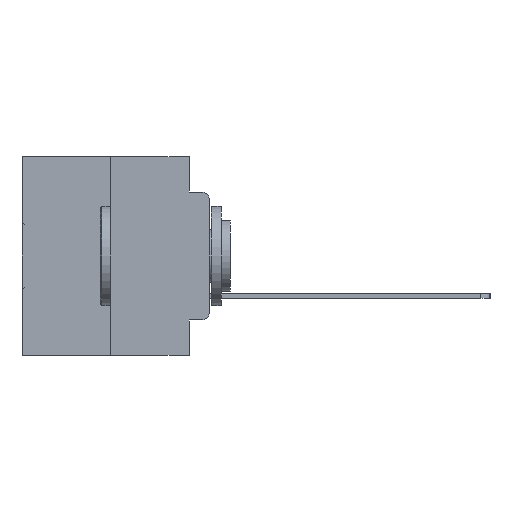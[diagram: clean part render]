
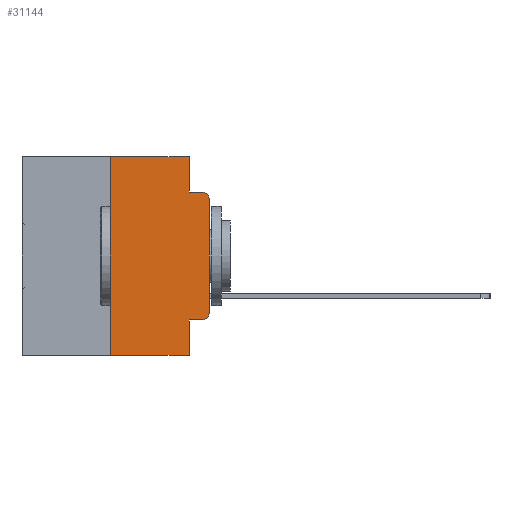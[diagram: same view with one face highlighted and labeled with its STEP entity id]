
A CAD part, left-side view. The second image highlights one B-rep face of the part: STEP entity #31144.
In plain terms, the highlighted planar face has unit normal (-1, 0, 0).
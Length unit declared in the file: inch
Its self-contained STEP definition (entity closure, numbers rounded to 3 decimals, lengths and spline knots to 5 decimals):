
#53 = LINE ( 'NONE', #8204, #6582 ) ;
#226 = CARTESIAN_POINT ( 'NONE',  ( 0., 0.051, -0.4115 ) ) ;
#747 = ORIENTED_EDGE ( 'NONE', *, *, #30713, .F. ) ;
#1232 = CARTESIAN_POINT ( 'NONE',  ( 0., 0.051, -0.0885 ) ) ;
#1269 = DIRECTION ( 'NONE',  ( 0., 0., -1. ) ) ;
#1496 = LINE ( 'NONE', #15368, #13036 ) ;
#2248 = ORIENTED_EDGE ( 'NONE', *, *, #18684, .T. ) ;
#2343 = CARTESIAN_POINT ( 'NONE',  ( 0., 0.02, -0.3915 ) ) ;
#2487 = VERTEX_POINT ( 'NONE', #26427 ) ;
#2679 = DIRECTION ( 'NONE',  ( 0., -1., 0. ) ) ;
#2840 = EDGE_CURVE ( 'NONE', #14777, #12980, #29415, .T. ) ;
#3729 = LINE ( 'NONE', #226, #22547 ) ;
#3903 = DIRECTION ( 'NONE',  ( 0., 0., -1. ) ) ;
#4452 = CARTESIAN_POINT ( 'NONE',  ( 0., 0.25, 0. ) ) ;
#4597 = DIRECTION ( 'NONE',  ( 0., 0., 1. ) ) ;
#4826 = DIRECTION ( 'NONE',  ( 0., 0., -1. ) ) ;
#5545 = EDGE_CURVE ( 'NONE', #18597, #29442, #30926, .T. ) ;
#5785 = ORIENTED_EDGE ( 'NONE', *, *, #19905, .T. ) ;
#6006 = VERTEX_POINT ( 'NONE', #20141 ) ;
#6008 = FACE_OUTER_BOUND ( 'NONE', #26589, .T. ) ;
#6169 = VERTEX_POINT ( 'NONE', #1232 ) ;
#6359 = LINE ( 'NONE', #21562, #18630 ) ;
#6582 = VECTOR ( 'NONE', #15618, 39.37008 ) ;
#6630 = AXIS2_PLACEMENT_3D ( 'NONE', #2343, #19522, #4826 ) ;
#6687 = VECTOR ( 'NONE', #18838, 39.37008 ) ;
#6896 = DIRECTION ( 'NONE',  ( 0., -1., 0. ) ) ;
#6928 = ORIENTED_EDGE ( 'NONE', *, *, #2840, .F. ) ;
#6996 = DIRECTION ( 'NONE',  ( 0., -1., 0. ) ) ;
#8204 = CARTESIAN_POINT ( 'NONE',  ( 0., 0.051, 0. ) ) ;
#8409 = EDGE_CURVE ( 'NONE', #2487, #21073, #9040, .T. ) ;
#8840 = ORIENTED_EDGE ( 'NONE', *, *, #9459, .F. ) ;
#9004 = CARTESIAN_POINT ( 'NONE',  ( 0., 0.473, 0. ) ) ;
#9040 = CIRCLE ( 'NONE', #6630, 0.02 ) ;
#9209 = ORIENTED_EDGE ( 'NONE', *, *, #5545, .T. ) ;
#9459 = EDGE_CURVE ( 'NONE', #28453, #6169, #18917, .T. ) ;
#10090 = CARTESIAN_POINT ( 'NONE',  ( 0., 0., -0.1085 ) ) ;
#11153 = DIRECTION ( 'NONE',  ( -1., 0., 0. ) ) ;
#12410 = VECTOR ( 'NONE', #3903, 39.37008 ) ;
#12980 = VERTEX_POINT ( 'NONE', #19435 ) ;
#13036 = VECTOR ( 'NONE', #27517, 39.37008 ) ;
#13221 = LINE ( 'NONE', #9004, #6687 ) ;
#13465 = ORIENTED_EDGE ( 'NONE', *, *, #30757, .T. ) ;
#14777 = VERTEX_POINT ( 'NONE', #15830 ) ;
#15368 = CARTESIAN_POINT ( 'NONE',  ( 0., 0., 0. ) ) ;
#15618 = DIRECTION ( 'NONE',  ( 0., 0., -1. ) ) ;
#15830 = CARTESIAN_POINT ( 'NONE',  ( 0., 0.25, -0.5 ) ) ;
#16004 = EDGE_CURVE ( 'NONE', #12980, #28453, #13221, .T. ) ;
#16005 = DIRECTION ( 'NONE',  ( 1., 0., 0. ) ) ;
#18221 = VERTEX_POINT ( 'NONE', #20937 ) ;
#18597 = VERTEX_POINT ( 'NONE', #10090 ) ;
#18630 = VECTOR ( 'NONE', #6896, 39.37008 ) ;
#18684 = EDGE_CURVE ( 'NONE', #21073, #18597, #1496, .T. ) ;
#18815 = ORIENTED_EDGE ( 'NONE', *, *, #8409, .T. ) ;
#18838 = DIRECTION ( 'NONE',  ( 0., -1., 0. ) ) ;
#18917 = LINE ( 'NONE', #25888, #12410 ) ;
#19435 = CARTESIAN_POINT ( 'NONE',  ( 0., 0.25, 0. ) ) ;
#19522 = DIRECTION ( 'NONE',  ( -1., 0., 0. ) ) ;
#19905 = EDGE_CURVE ( 'NONE', #18221, #2487, #3729, .T. ) ;
#20141 = CARTESIAN_POINT ( 'NONE',  ( 0., 0.051, -0.5 ) ) ;
#20735 = ORIENTED_EDGE ( 'NONE', *, *, #26474, .F. ) ;
#20937 = CARTESIAN_POINT ( 'NONE',  ( 0., 0.051, -0.4115 ) ) ;
#21073 = VERTEX_POINT ( 'NONE', #21825 ) ;
#21562 = CARTESIAN_POINT ( 'NONE',  ( 0., 0.051, -0.0885 ) ) ;
#21825 = CARTESIAN_POINT ( 'NONE',  ( 0., 0., -0.3915 ) ) ;
#22281 = CARTESIAN_POINT ( 'NONE',  ( 0., 0.02, -0.0885 ) ) ;
#22547 = VECTOR ( 'NONE', #2679, 39.37008 ) ;
#22764 = CARTESIAN_POINT ( 'NONE',  ( 0., 0.051, 0. ) ) ;
#22968 = VECTOR ( 'NONE', #4597, 39.37008 ) ;
#24146 = CARTESIAN_POINT ( 'NONE',  ( 0., 0.473, -0.5 ) ) ;
#24244 = AXIS2_PLACEMENT_3D ( 'NONE', #25834, #11153, #28249 ) ;
#24400 = LINE ( 'NONE', #24146, #31560 ) ;
#25272 = AXIS2_PLACEMENT_3D ( 'NONE', #30565, #16005, #1269 ) ;
#25834 = CARTESIAN_POINT ( 'NONE',  ( 0., 0.02, -0.1085 ) ) ;
#25888 = CARTESIAN_POINT ( 'NONE',  ( 0., 0.051, 0. ) ) ;
#26427 = CARTESIAN_POINT ( 'NONE',  ( 0., 0.02, -0.4115 ) ) ;
#26474 = EDGE_CURVE ( 'NONE', #18221, #6006, #53, .T. ) ;
#26589 = EDGE_LOOP ( 'NONE', ( #2248, #9209, #747, #8840, #30607, #6928, #13465, #20735, #5785, #18815 ) ) ;
#27517 = DIRECTION ( 'NONE',  ( 0., 0., 1. ) ) ;
#28141 = PLANE ( 'NONE',  #25272 ) ;
#28249 = DIRECTION ( 'NONE',  ( 0., 0., -1. ) ) ;
#28453 = VERTEX_POINT ( 'NONE', #22764 ) ;
#29415 = LINE ( 'NONE', #4452, #22968 ) ;
#29442 = VERTEX_POINT ( 'NONE', #22281 ) ;
#30565 = CARTESIAN_POINT ( 'NONE',  ( 0., 0.473, 0. ) ) ;
#30607 = ORIENTED_EDGE ( 'NONE', *, *, #16004, .F. ) ;
#30713 = EDGE_CURVE ( 'NONE', #6169, #29442, #6359, .T. ) ;
#30757 = EDGE_CURVE ( 'NONE', #14777, #6006, #24400, .T. ) ;
#30926 = CIRCLE ( 'NONE', #24244, 0.02 ) ;
#31144 = ADVANCED_FACE ( 'NONE', ( #6008 ), #28141, .F. ) ;
#31560 = VECTOR ( 'NONE', #6996, 39.37008 ) ;
